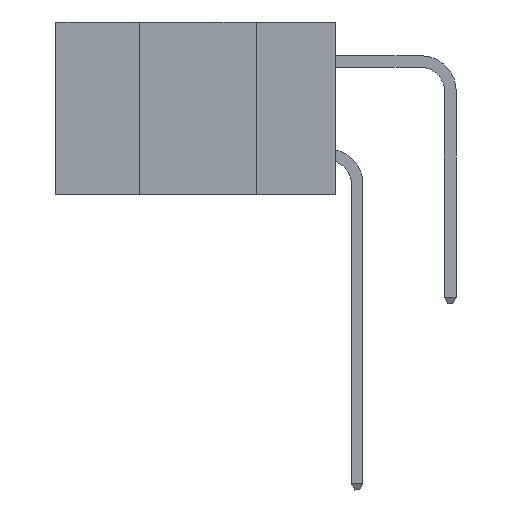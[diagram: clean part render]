
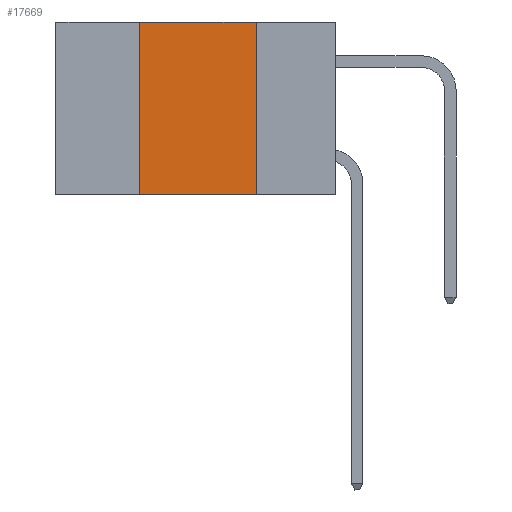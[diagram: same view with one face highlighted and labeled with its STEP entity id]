
A CAD part, left-side view. The second image highlights one B-rep face of the part: STEP entity #17669.
In plain terms, the highlighted planar face has unit normal (-1, 0, 0).
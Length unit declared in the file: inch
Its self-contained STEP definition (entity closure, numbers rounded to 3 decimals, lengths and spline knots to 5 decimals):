
#1845 = LINE ( 'NONE', #21503, #8332 ) ;
#2142 = EDGE_LOOP ( 'NONE', ( #26843, #28525, #15806, #23080 ) ) ;
#3002 = FACE_OUTER_BOUND ( 'NONE', #2142, .T. ) ;
#3077 = CARTESIAN_POINT ( 'NONE',  ( 0., 0.17, 0. ) ) ;
#3242 = CARTESIAN_POINT ( 'NONE',  ( 0., 0.42, 0. ) ) ;
#3521 = VERTEX_POINT ( 'NONE', #3077 ) ;
#6497 = CARTESIAN_POINT ( 'NONE',  ( 0., 0.17, -0.37 ) ) ;
#7851 = DIRECTION ( 'NONE',  ( 0., -1., 0. ) ) ;
#7934 = DIRECTION ( 'NONE',  ( 0., -1., 0. ) ) ;
#8332 = VECTOR ( 'NONE', #7934, 39.37008 ) ;
#9410 = VECTOR ( 'NONE', #14402, 39.37008 ) ;
#9760 = CARTESIAN_POINT ( 'NONE',  ( 0., 0.6, 0. ) ) ;
#11406 = DIRECTION ( 'NONE',  ( 0., 0., 1. ) ) ;
#12495 = DIRECTION ( 'NONE',  ( 0., 0., -1. ) ) ;
#14402 = DIRECTION ( 'NONE',  ( 0., 0., -1. ) ) ;
#14949 = VECTOR ( 'NONE', #11406, 39.37008 ) ;
#15806 = ORIENTED_EDGE ( 'NONE', *, *, #25051, .F. ) ;
#17669 = ADVANCED_FACE ( 'NONE', ( #3002 ), #20613, .F. ) ;
#20613 = PLANE ( 'NONE',  #30427 ) ;
#21503 = CARTESIAN_POINT ( 'NONE',  ( 0., 0.6, -0.37 ) ) ;
#22085 = EDGE_CURVE ( 'NONE', #26878, #32289, #1845, .T. ) ;
#22894 = VECTOR ( 'NONE', #7851, 39.37008 ) ;
#23080 = ORIENTED_EDGE ( 'NONE', *, *, #22085, .T. ) ;
#23922 = LINE ( 'NONE', #30650, #9410 ) ;
#25051 = EDGE_CURVE ( 'NONE', #26878, #30970, #29355, .T. ) ;
#26843 = ORIENTED_EDGE ( 'NONE', *, *, #34683, .F. ) ;
#26878 = VERTEX_POINT ( 'NONE', #33032 ) ;
#28525 = ORIENTED_EDGE ( 'NONE', *, *, #31435, .F. ) ;
#28758 = DIRECTION ( 'NONE',  ( 1., 0., 0. ) ) ;
#29355 = LINE ( 'NONE', #3242, #14949 ) ;
#29450 = CARTESIAN_POINT ( 'NONE',  ( 0., 0.6, 0. ) ) ;
#30427 = AXIS2_PLACEMENT_3D ( 'NONE', #9760, #28758, #12495 ) ;
#30650 = CARTESIAN_POINT ( 'NONE',  ( 0., 0.17, 0. ) ) ;
#30903 = LINE ( 'NONE', #29450, #22894 ) ;
#30970 = VERTEX_POINT ( 'NONE', #33116 ) ;
#31435 = EDGE_CURVE ( 'NONE', #30970, #3521, #30903, .T. ) ;
#32289 = VERTEX_POINT ( 'NONE', #6497 ) ;
#33032 = CARTESIAN_POINT ( 'NONE',  ( 0., 0.42, -0.37 ) ) ;
#33116 = CARTESIAN_POINT ( 'NONE',  ( 0., 0.42, 0. ) ) ;
#34683 = EDGE_CURVE ( 'NONE', #3521, #32289, #23922, .T. ) ;
